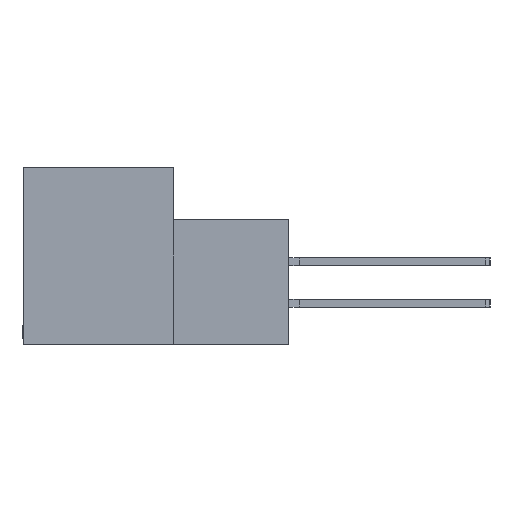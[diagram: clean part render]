
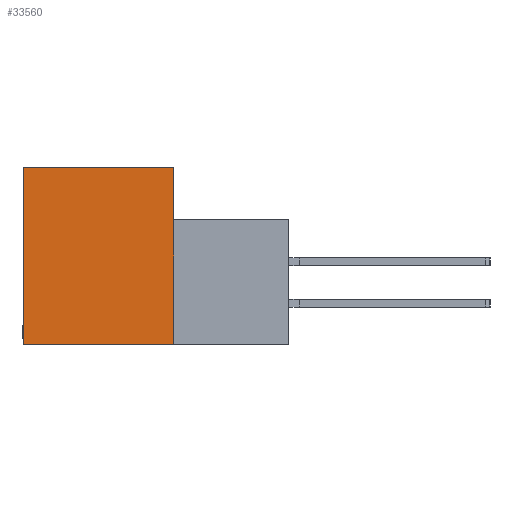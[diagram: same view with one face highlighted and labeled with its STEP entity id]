
A CAD part, left-side view. The second image highlights one B-rep face of the part: STEP entity #33560.
In plain terms, the highlighted planar face has unit normal (-1, 0, 0).
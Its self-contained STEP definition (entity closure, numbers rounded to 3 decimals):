
#1283 = PLANE ( 'NONE',  #32573 ) ;
#1878 = EDGE_LOOP ( 'NONE', ( #17329, #19584, #26252, #45592 ) ) ;
#4253 = FACE_OUTER_BOUND ( 'NONE', #1878, .T. ) ;
#4411 = VECTOR ( 'NONE', #27365, 1000. ) ;
#4869 = DIRECTION ( 'NONE',  ( 1., 0., 0. ) ) ;
#5379 = LINE ( 'NONE', #30772, #11983 ) ;
#5389 = VERTEX_POINT ( 'NONE', #19329 ) ;
#6115 = VECTOR ( 'NONE', #22176, 1000. ) ;
#7133 = CARTESIAN_POINT ( 'NONE',  ( 0., 11.506, 0. ) ) ;
#7976 = CARTESIAN_POINT ( 'NONE',  ( 0., 0., 0. ) ) ;
#8412 = DIRECTION ( 'NONE',  ( 0., 0., -1. ) ) ;
#11971 = CARTESIAN_POINT ( 'NONE',  ( 0., 0., 0. ) ) ;
#11983 = VECTOR ( 'NONE', #16165, 1000. ) ;
#12633 = EDGE_CURVE ( 'NONE', #18536, #5389, #26034, .T. ) ;
#12689 = LINE ( 'NONE', #31040, #4411 ) ;
#13872 = EDGE_CURVE ( 'NONE', #25233, #29445, #35268, .T. ) ;
#14333 = VECTOR ( 'NONE', #20772, 1000. ) ;
#16165 = DIRECTION ( 'NONE',  ( 0., 1., 0. ) ) ;
#17248 = CARTESIAN_POINT ( 'NONE',  ( 0., 11.506, -13.487 ) ) ;
#17329 = ORIENTED_EDGE ( 'NONE', *, *, #39599, .F. ) ;
#18536 = VERTEX_POINT ( 'NONE', #24723 ) ;
#19329 = CARTESIAN_POINT ( 'NONE',  ( 0., 0., -13.487 ) ) ;
#19584 = ORIENTED_EDGE ( 'NONE', *, *, #12633, .F. ) ;
#20772 = DIRECTION ( 'NONE',  ( 0., 0., 1. ) ) ;
#22176 = DIRECTION ( 'NONE',  ( 0., 0., -1. ) ) ;
#23179 = EDGE_CURVE ( 'NONE', #29445, #18536, #12689, .T. ) ;
#24723 = CARTESIAN_POINT ( 'NONE',  ( 0., 0., 0. ) ) ;
#25233 = VERTEX_POINT ( 'NONE', #34706 ) ;
#26034 = LINE ( 'NONE', #7976, #6115 ) ;
#26252 = ORIENTED_EDGE ( 'NONE', *, *, #23179, .F. ) ;
#27365 = DIRECTION ( 'NONE',  ( 0., -1., 0. ) ) ;
#29445 = VERTEX_POINT ( 'NONE', #7133 ) ;
#30772 = CARTESIAN_POINT ( 'NONE',  ( 0., -8.814, -13.487 ) ) ;
#31040 = CARTESIAN_POINT ( 'NONE',  ( 0., 11.506, 0. ) ) ;
#32573 = AXIS2_PLACEMENT_3D ( 'NONE', #11971, #4869, #8412 ) ;
#33560 = ADVANCED_FACE ( 'NONE', ( #4253 ), #1283, .F. ) ;
#34706 = CARTESIAN_POINT ( 'NONE',  ( 0., 11.506, -13.487 ) ) ;
#35268 = LINE ( 'NONE', #17248, #14333 ) ;
#39599 = EDGE_CURVE ( 'NONE', #5389, #25233, #5379, .T. ) ;
#45592 = ORIENTED_EDGE ( 'NONE', *, *, #13872, .F. ) ;
